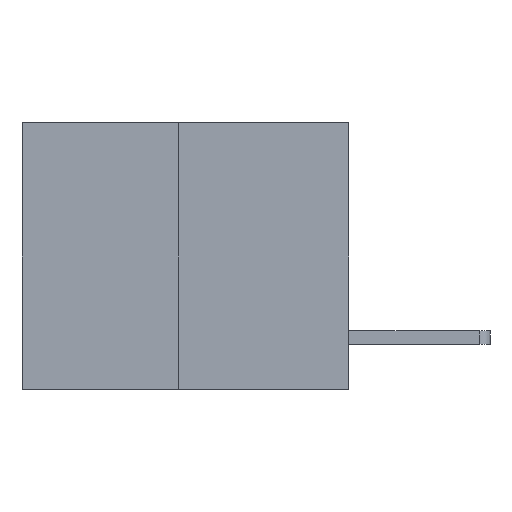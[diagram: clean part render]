
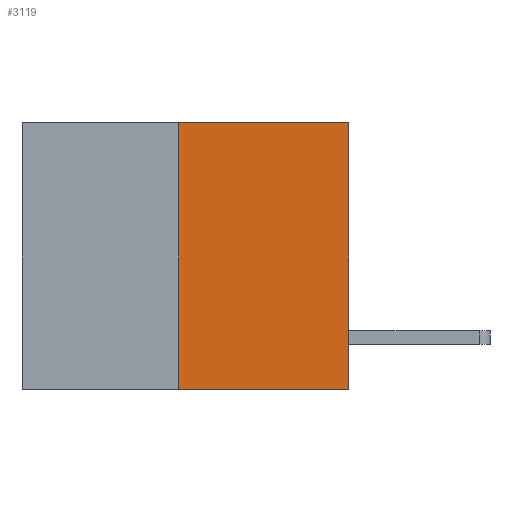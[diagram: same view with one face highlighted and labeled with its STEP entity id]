
A CAD part, left-side view. The second image highlights one B-rep face of the part: STEP entity #3119.
In plain terms, the highlighted planar face has unit normal (-1, 0, 0).
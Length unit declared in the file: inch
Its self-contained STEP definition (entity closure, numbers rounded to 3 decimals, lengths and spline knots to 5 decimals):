
#224 = DIRECTION ( 'NONE',  ( 0., -1., 0. ) ) ;
#278 = ORIENTED_EDGE ( 'NONE', *, *, #8459, .T. ) ;
#324 = DIRECTION ( 'NONE',  ( 0., 0., 1. ) ) ;
#569 = DIRECTION ( 'NONE',  ( 0., 0., 1. ) ) ;
#1195 = DIRECTION ( 'NONE',  ( 0., -1., 0. ) ) ;
#1209 = DIRECTION ( 'NONE',  ( 0., 0., -1. ) ) ;
#1462 = VERTEX_POINT ( 'NONE', #1763 ) ;
#1512 = VECTOR ( 'NONE', #1195, 39.37008 ) ;
#1516 = EDGE_CURVE ( 'NONE', #4544, #9211, #3210, .T. ) ;
#1631 = CARTESIAN_POINT ( 'NONE',  ( 0., 0., 0. ) ) ;
#1763 = CARTESIAN_POINT ( 'NONE',  ( 0., 0.312, 0. ) ) ;
#2119 = CARTESIAN_POINT ( 'NONE',  ( 0., 0., -0.49 ) ) ;
#2127 = EDGE_LOOP ( 'NONE', ( #4293, #4401, #278, #5317 ) ) ;
#2168 = CARTESIAN_POINT ( 'NONE',  ( 0., 0., 0. ) ) ;
#2191 = LINE ( 'NONE', #2168, #3568 ) ;
#3119 = ADVANCED_FACE ( 'NONE', ( #5234 ), #5580, .F. ) ;
#3210 = LINE ( 'NONE', #3877, #5488 ) ;
#3387 = VERTEX_POINT ( 'NONE', #1631 ) ;
#3568 = VECTOR ( 'NONE', #569, 39.37008 ) ;
#3793 = LINE ( 'NONE', #8520, #1512 ) ;
#3877 = CARTESIAN_POINT ( 'NONE',  ( 0., 0.6, -0.49 ) ) ;
#4293 = ORIENTED_EDGE ( 'NONE', *, *, #8107, .F. ) ;
#4401 = ORIENTED_EDGE ( 'NONE', *, *, #1516, .T. ) ;
#4544 = VERTEX_POINT ( 'NONE', #5811 ) ;
#5234 = FACE_OUTER_BOUND ( 'NONE', #2127, .T. ) ;
#5317 = ORIENTED_EDGE ( 'NONE', *, *, #8341, .F. ) ;
#5488 = VECTOR ( 'NONE', #224, 39.37008 ) ;
#5580 = PLANE ( 'NONE',  #5775 ) ;
#5775 = AXIS2_PLACEMENT_3D ( 'NONE', #6321, #9336, #1209 ) ;
#5811 = CARTESIAN_POINT ( 'NONE',  ( 0., 0.312, -0.49 ) ) ;
#6321 = CARTESIAN_POINT ( 'NONE',  ( 0., 0.6, 0. ) ) ;
#8107 = EDGE_CURVE ( 'NONE', #4544, #1462, #8338, .T. ) ;
#8224 = VECTOR ( 'NONE', #324, 39.37008 ) ;
#8338 = LINE ( 'NONE', #9048, #8224 ) ;
#8341 = EDGE_CURVE ( 'NONE', #1462, #3387, #3793, .T. ) ;
#8459 = EDGE_CURVE ( 'NONE', #9211, #3387, #2191, .T. ) ;
#8520 = CARTESIAN_POINT ( 'NONE',  ( 0., 0.6, 0. ) ) ;
#9048 = CARTESIAN_POINT ( 'NONE',  ( 0., 0.312, -0.49 ) ) ;
#9211 = VERTEX_POINT ( 'NONE', #2119 ) ;
#9336 = DIRECTION ( 'NONE',  ( 1., 0., 0. ) ) ;
